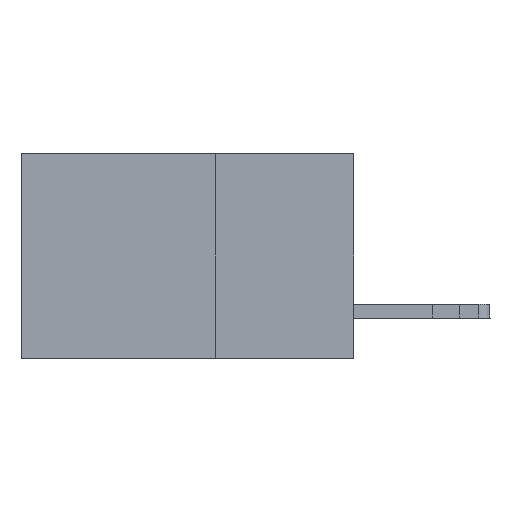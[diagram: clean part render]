
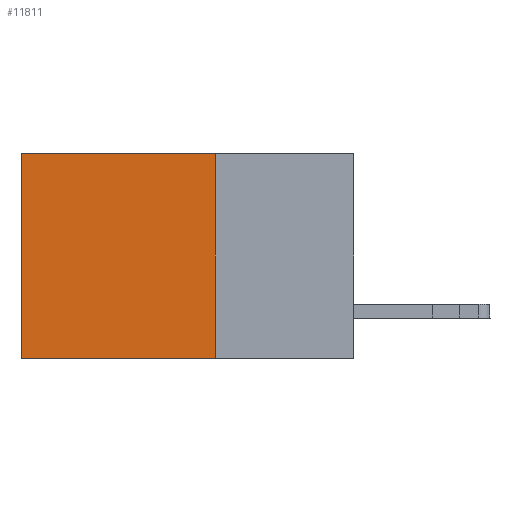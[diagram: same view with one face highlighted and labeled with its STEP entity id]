
A CAD part, left-side view. The second image highlights one B-rep face of the part: STEP entity #11811.
In plain terms, the highlighted planar face has unit normal (-1, 0, 0).
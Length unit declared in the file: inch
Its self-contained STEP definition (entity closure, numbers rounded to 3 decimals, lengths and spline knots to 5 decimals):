
#754 = EDGE_CURVE ( 'NONE', #17470, #17058, #4394, .T. ) ;
#863 = EDGE_CURVE ( 'NONE', #19727, #14233, #3015, .T. ) ;
#899 = FACE_OUTER_BOUND ( 'NONE', #19843, .T. ) ;
#1423 = DIRECTION ( 'NONE',  ( 0., 0., -1. ) ) ;
#1693 = DIRECTION ( 'NONE',  ( 0., 1., 0. ) ) ;
#2047 = LINE ( 'NONE', #13043, #12465 ) ;
#2726 = VECTOR ( 'NONE', #1423, 39.37008 ) ;
#2842 = CARTESIAN_POINT ( 'NONE',  ( 0.2875, 0.25, 0. ) ) ;
#3015 = LINE ( 'NONE', #8993, #2726 ) ;
#4394 = LINE ( 'NONE', #11720, #13261 ) ;
#7559 = LINE ( 'NONE', #14771, #23276 ) ;
#8993 = CARTESIAN_POINT ( 'NONE',  ( 0.2875, 0.25, 0. ) ) ;
#9467 = EDGE_CURVE ( 'NONE', #14233, #17058, #2047, .T. ) ;
#10281 = ORIENTED_EDGE ( 'NONE', *, *, #863, .F. ) ;
#10293 = DIRECTION ( 'NONE',  ( 0., 0., -1. ) ) ;
#10538 = DIRECTION ( 'NONE',  ( 1., 0., 0. ) ) ;
#11253 = ORIENTED_EDGE ( 'NONE', *, *, #9467, .F. ) ;
#11720 = CARTESIAN_POINT ( 'NONE',  ( 0.2875, 0.6, 0. ) ) ;
#11811 = ADVANCED_FACE ( 'NONE', ( #899 ), #23113, .F. ) ;
#12465 = VECTOR ( 'NONE', #15004, 39.37008 ) ;
#12768 = ORIENTED_EDGE ( 'NONE', *, *, #22875, .T. ) ;
#13043 = CARTESIAN_POINT ( 'NONE',  ( 0.2875, 0.25, -0.37 ) ) ;
#13261 = VECTOR ( 'NONE', #22707, 39.37008 ) ;
#14233 = VERTEX_POINT ( 'NONE', #23038 ) ;
#14771 = CARTESIAN_POINT ( 'NONE',  ( 0.2875, 0.25, 0. ) ) ;
#14798 = AXIS2_PLACEMENT_3D ( 'NONE', #2842, #10538, #10293 ) ;
#15004 = DIRECTION ( 'NONE',  ( 0., 1., 0. ) ) ;
#16566 = CARTESIAN_POINT ( 'NONE',  ( 0.2875, 0.6, 0. ) ) ;
#17058 = VERTEX_POINT ( 'NONE', #20132 ) ;
#17470 = VERTEX_POINT ( 'NONE', #16566 ) ;
#19727 = VERTEX_POINT ( 'NONE', #19983 ) ;
#19843 = EDGE_LOOP ( 'NONE', ( #20897, #11253, #10281, #12768 ) ) ;
#19983 = CARTESIAN_POINT ( 'NONE',  ( 0.2875, 0.25, 0. ) ) ;
#20132 = CARTESIAN_POINT ( 'NONE',  ( 0.2875, 0.6, -0.37 ) ) ;
#20897 = ORIENTED_EDGE ( 'NONE', *, *, #754, .T. ) ;
#22707 = DIRECTION ( 'NONE',  ( 0., 0., -1. ) ) ;
#22875 = EDGE_CURVE ( 'NONE', #19727, #17470, #7559, .T. ) ;
#23038 = CARTESIAN_POINT ( 'NONE',  ( 0.2875, 0.25, -0.37 ) ) ;
#23113 = PLANE ( 'NONE',  #14798 ) ;
#23276 = VECTOR ( 'NONE', #1693, 39.37008 ) ;
